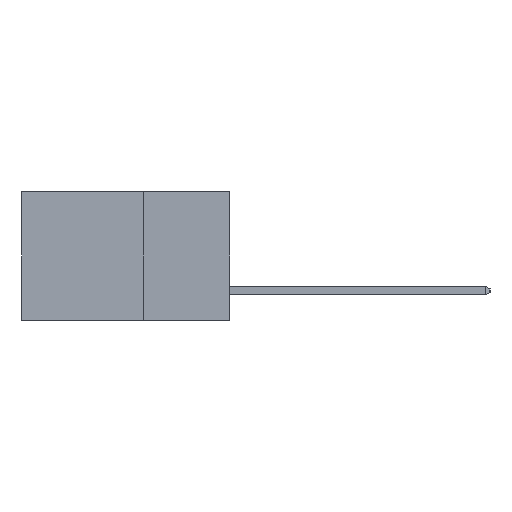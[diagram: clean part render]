
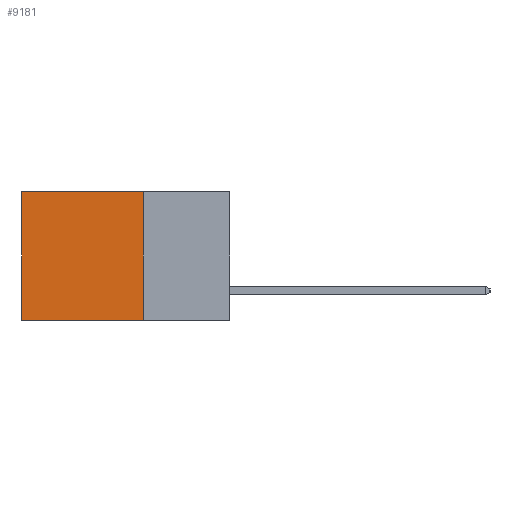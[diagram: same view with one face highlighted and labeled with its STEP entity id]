
A CAD part, left-side view. The second image highlights one B-rep face of the part: STEP entity #9181.
In plain terms, the highlighted planar face has unit normal (-1, 0, 0).
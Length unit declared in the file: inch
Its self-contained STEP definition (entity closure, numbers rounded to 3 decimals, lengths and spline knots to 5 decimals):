
#648 = FACE_OUTER_BOUND ( 'NONE', #5947, .T. ) ;
#1095 = LINE ( 'NONE', #18391, #1587 ) ;
#1547 = ORIENTED_EDGE ( 'NONE', *, *, #9924, .T. ) ;
#1587 = VECTOR ( 'NONE', #11029, 39.37008 ) ;
#2010 = VECTOR ( 'NONE', #16534, 39.37008 ) ;
#2100 = EDGE_CURVE ( 'NONE', #15471, #16081, #10407, .T. ) ;
#3365 = ORIENTED_EDGE ( 'NONE', *, *, #16924, .F. ) ;
#3826 = VECTOR ( 'NONE', #4585, 39.37008 ) ;
#4515 = CARTESIAN_POINT ( 'NONE',  ( 0.298, 0.25, 0. ) ) ;
#4585 = DIRECTION ( 'NONE',  ( 0., 0., -1. ) ) ;
#5947 = EDGE_LOOP ( 'NONE', ( #1547, #3365, #18055, #17666 ) ) ;
#6380 = VERTEX_POINT ( 'NONE', #11330 ) ;
#6411 = VECTOR ( 'NONE', #15786, 39.37008 ) ;
#7473 = CARTESIAN_POINT ( 'NONE',  ( 0.298, 0.25, 0. ) ) ;
#8322 = VERTEX_POINT ( 'NONE', #8906 ) ;
#8903 = DIRECTION ( 'NONE',  ( 1., 0., 0. ) ) ;
#8906 = CARTESIAN_POINT ( 'NONE',  ( 0.298, 0.6, 0. ) ) ;
#9181 = ADVANCED_FACE ( 'NONE', ( #648 ), #16425, .F. ) ;
#9924 = EDGE_CURVE ( 'NONE', #8322, #6380, #12302, .T. ) ;
#10407 = LINE ( 'NONE', #17498, #6411 ) ;
#10445 = CARTESIAN_POINT ( 'NONE',  ( 0.298, 0.25, -0.37 ) ) ;
#11029 = DIRECTION ( 'NONE',  ( 0., 1., 0. ) ) ;
#11330 = CARTESIAN_POINT ( 'NONE',  ( 0.298, 0.6, -0.37 ) ) ;
#12083 = CARTESIAN_POINT ( 'NONE',  ( 0.298, 0.6, 0. ) ) ;
#12302 = LINE ( 'NONE', #12083, #3826 ) ;
#12783 = EDGE_CURVE ( 'NONE', #15471, #8322, #18464, .T. ) ;
#13255 = AXIS2_PLACEMENT_3D ( 'NONE', #17897, #8903, #19366 ) ;
#15471 = VERTEX_POINT ( 'NONE', #7473 ) ;
#15786 = DIRECTION ( 'NONE',  ( 0., 0., -1. ) ) ;
#16081 = VERTEX_POINT ( 'NONE', #10445 ) ;
#16425 = PLANE ( 'NONE',  #13255 ) ;
#16534 = DIRECTION ( 'NONE',  ( 0., 1., 0. ) ) ;
#16924 = EDGE_CURVE ( 'NONE', #16081, #6380, #1095, .T. ) ;
#17498 = CARTESIAN_POINT ( 'NONE',  ( 0.298, 0.25, 0. ) ) ;
#17666 = ORIENTED_EDGE ( 'NONE', *, *, #12783, .T. ) ;
#17897 = CARTESIAN_POINT ( 'NONE',  ( 0.298, 0.25, 0. ) ) ;
#18055 = ORIENTED_EDGE ( 'NONE', *, *, #2100, .F. ) ;
#18391 = CARTESIAN_POINT ( 'NONE',  ( 0.298, 0.25, -0.37 ) ) ;
#18464 = LINE ( 'NONE', #4515, #2010 ) ;
#19366 = DIRECTION ( 'NONE',  ( 0., 0., -1. ) ) ;
